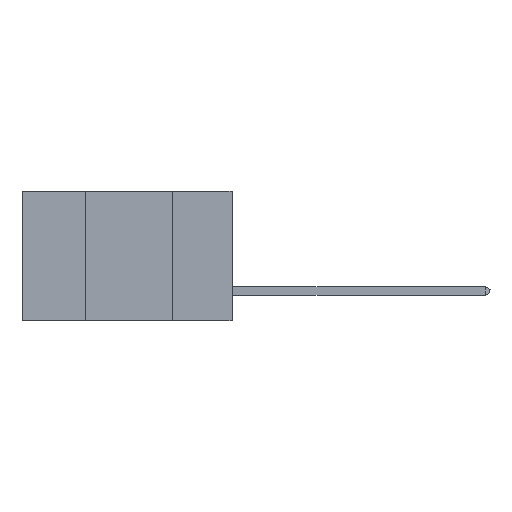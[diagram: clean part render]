
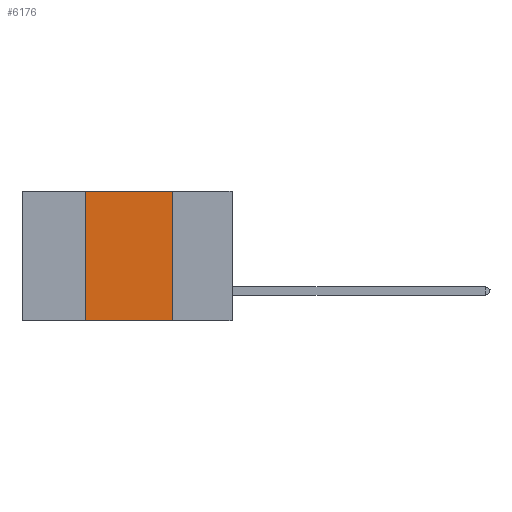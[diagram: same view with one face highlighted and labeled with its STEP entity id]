
A CAD part, left-side view. The second image highlights one B-rep face of the part: STEP entity #6176.
In plain terms, the highlighted planar face has unit normal (-1, 0, 0).
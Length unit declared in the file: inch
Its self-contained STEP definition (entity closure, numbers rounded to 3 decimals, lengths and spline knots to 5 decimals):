
#776 = EDGE_LOOP ( 'NONE', ( #1675, #2551, #19173, #1209 ) ) ;
#1209 = ORIENTED_EDGE ( 'NONE', *, *, #11546, .T. ) ;
#1484 = CARTESIAN_POINT ( 'NONE',  ( 0., 0.6, 0. ) ) ;
#1675 = ORIENTED_EDGE ( 'NONE', *, *, #15679, .F. ) ;
#1717 = DIRECTION ( 'NONE',  ( 0., -1., 0. ) ) ;
#2542 = CARTESIAN_POINT ( 'NONE',  ( 0., 0.42, 0. ) ) ;
#2551 = ORIENTED_EDGE ( 'NONE', *, *, #9204, .F. ) ;
#5122 = CARTESIAN_POINT ( 'NONE',  ( 0., 0.6, 0. ) ) ;
#6176 = ADVANCED_FACE ( 'NONE', ( #10755 ), #24471, .F. ) ;
#7427 = VERTEX_POINT ( 'NONE', #8486 ) ;
#8049 = EDGE_CURVE ( 'NONE', #21747, #12552, #13956, .T. ) ;
#8486 = CARTESIAN_POINT ( 'NONE',  ( 0., 0.17, 0. ) ) ;
#9070 = DIRECTION ( 'NONE',  ( 0., -1., 0. ) ) ;
#9204 = EDGE_CURVE ( 'NONE', #12552, #7427, #13286, .T. ) ;
#10143 = VECTOR ( 'NONE', #24527, 39.37008 ) ;
#10755 = FACE_OUTER_BOUND ( 'NONE', #776, .T. ) ;
#11054 = DIRECTION ( 'NONE',  ( 0., 0., -1. ) ) ;
#11546 = EDGE_CURVE ( 'NONE', #21747, #12701, #17348, .T. ) ;
#11639 = VECTOR ( 'NONE', #1717, 39.37008 ) ;
#12552 = VERTEX_POINT ( 'NONE', #17025 ) ;
#12701 = VERTEX_POINT ( 'NONE', #20591 ) ;
#12802 = CARTESIAN_POINT ( 'NONE',  ( 0., 0.17, 0. ) ) ;
#13061 = VECTOR ( 'NONE', #22051, 39.37008 ) ;
#13286 = LINE ( 'NONE', #5122, #16308 ) ;
#13956 = LINE ( 'NONE', #2542, #13061 ) ;
#15679 = EDGE_CURVE ( 'NONE', #7427, #12701, #23406, .T. ) ;
#16087 = CARTESIAN_POINT ( 'NONE',  ( 0., 0.42, -0.37 ) ) ;
#16308 = VECTOR ( 'NONE', #9070, 39.37008 ) ;
#17025 = CARTESIAN_POINT ( 'NONE',  ( 0., 0.42, 0. ) ) ;
#17348 = LINE ( 'NONE', #21022, #11639 ) ;
#17845 = AXIS2_PLACEMENT_3D ( 'NONE', #1484, #24714, #11054 ) ;
#19173 = ORIENTED_EDGE ( 'NONE', *, *, #8049, .F. ) ;
#20591 = CARTESIAN_POINT ( 'NONE',  ( 0., 0.17, -0.37 ) ) ;
#21022 = CARTESIAN_POINT ( 'NONE',  ( 0., 0.6, -0.37 ) ) ;
#21747 = VERTEX_POINT ( 'NONE', #16087 ) ;
#22051 = DIRECTION ( 'NONE',  ( 0., 0., 1. ) ) ;
#23406 = LINE ( 'NONE', #12802, #10143 ) ;
#24471 = PLANE ( 'NONE',  #17845 ) ;
#24527 = DIRECTION ( 'NONE',  ( 0., 0., -1. ) ) ;
#24714 = DIRECTION ( 'NONE',  ( 1., 0., 0. ) ) ;
